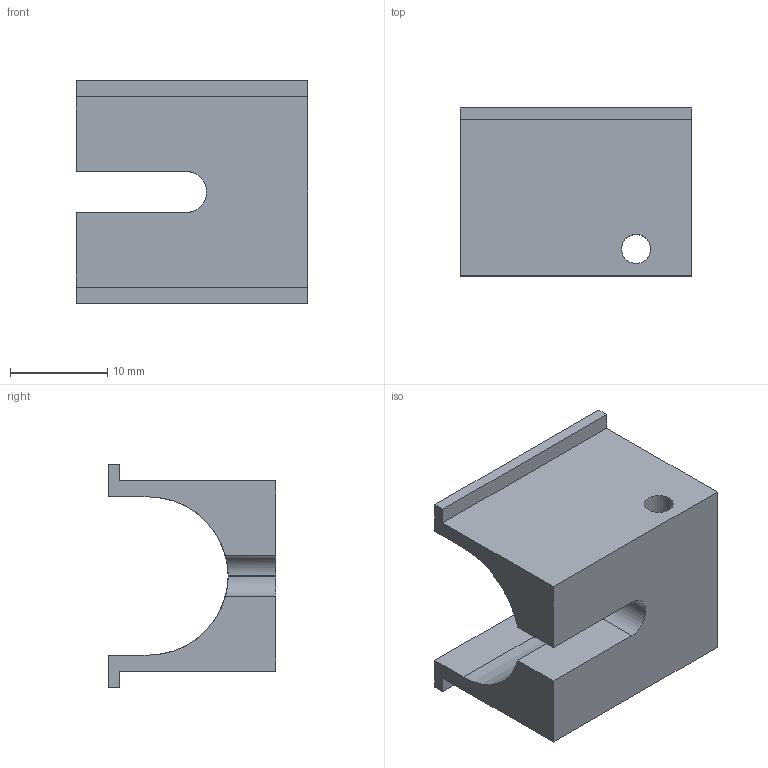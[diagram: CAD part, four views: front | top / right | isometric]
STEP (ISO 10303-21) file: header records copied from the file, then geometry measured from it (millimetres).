
FILE_DESCRIPTION(/* description */ (''),/* implementation_level */ '2;1');
FILE_NAME(/* name */ 'Front Rail Block.stp',/* time_stamp */ '2019-03-17T16:28:10-05:00',/* author */ ('johne'),/* organization */ (''),/* preprocessor_version */ 'ST-DEVELOPER v16.13',/* originating_system */ 'Autodesk Inventor 2018',/* authorisation */ '');
FILE_SCHEMA (('AUTOMOTIVE_DESIGN { 1 0 10303 214 3 1 1 }'));
Length unit declared in the file: millimetre
Products named in the file (1): Component1
Bounding box: 23.86 x 17.25 x 23 mm (x, y, z)
Volume: 3627.4 mm3; surface area: 2871.8 mm2
Topology: 1 solids, 1 shells, 21 faces, 57 edges, 38 vertices
Faces by surface type: plane 17, cylinder 4
Full cylindrical faces by diameter (mm): 3 x1
Entity records: 705 total; most frequent: CARTESIAN_POINT 134, ORIENTED_EDGE 112, DIRECTION 106, EDGE_CURVE 56, LINE 46, VECTOR 46, VERTEX_POINT 38, AXIS2_PLACEMENT_3D 30
